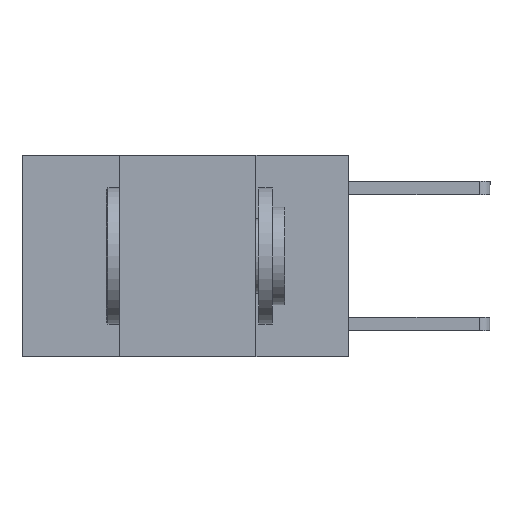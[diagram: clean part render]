
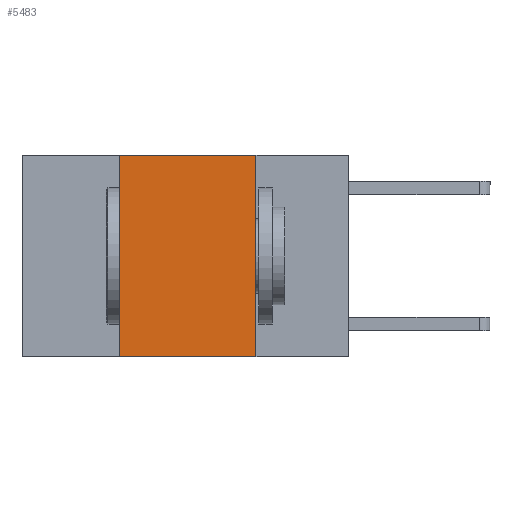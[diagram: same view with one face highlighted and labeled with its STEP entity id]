
A CAD part, left-side view. The second image highlights one B-rep face of the part: STEP entity #5483.
In plain terms, the highlighted planar face has unit normal (-1, 0, 0).
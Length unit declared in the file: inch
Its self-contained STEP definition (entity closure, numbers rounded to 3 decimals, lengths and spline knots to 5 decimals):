
#61 = ORIENTED_EDGE ( 'NONE', *, *, #5642, .F. ) ;
#530 = DIRECTION ( 'NONE',  ( 0., 0., -1. ) ) ;
#706 = LINE ( 'NONE', #3466, #3795 ) ;
#716 = CARTESIAN_POINT ( 'NONE',  ( 0., 0.42, 0. ) ) ;
#812 = VERTEX_POINT ( 'NONE', #1361 ) ;
#1120 = CARTESIAN_POINT ( 'NONE',  ( 0., 0.17, -0.37 ) ) ;
#1247 = LINE ( 'NONE', #4108, #3077 ) ;
#1333 = AXIS2_PLACEMENT_3D ( 'NONE', #3973, #8892, #530 ) ;
#1361 = CARTESIAN_POINT ( 'NONE',  ( 0., 0.42, -0.37 ) ) ;
#1599 = ORIENTED_EDGE ( 'NONE', *, *, #5420, .F. ) ;
#1929 = LINE ( 'NONE', #4697, #6848 ) ;
#2064 = VERTEX_POINT ( 'NONE', #1120 ) ;
#2792 = DIRECTION ( 'NONE',  ( 0., -1., 0. ) ) ;
#3077 = VECTOR ( 'NONE', #4789, 39.37008 ) ;
#3298 = CARTESIAN_POINT ( 'NONE',  ( 0., 0.17, 0. ) ) ;
#3466 = CARTESIAN_POINT ( 'NONE',  ( 0., 0.6, -0.37 ) ) ;
#3509 = LINE ( 'NONE', #5690, #5982 ) ;
#3795 = VECTOR ( 'NONE', #2792, 39.37008 ) ;
#3973 = CARTESIAN_POINT ( 'NONE',  ( 0., 0.6, 0. ) ) ;
#4108 = CARTESIAN_POINT ( 'NONE',  ( 0., 0.17, 0. ) ) ;
#4154 = DIRECTION ( 'NONE',  ( 0., -1., 0. ) ) ;
#4661 = FACE_OUTER_BOUND ( 'NONE', #7631, .T. ) ;
#4697 = CARTESIAN_POINT ( 'NONE',  ( 0., 0.42, 0. ) ) ;
#4789 = DIRECTION ( 'NONE',  ( 0., 0., -1. ) ) ;
#4960 = ORIENTED_EDGE ( 'NONE', *, *, #5509, .F. ) ;
#5420 = EDGE_CURVE ( 'NONE', #7531, #2064, #1247, .T. ) ;
#5483 = ADVANCED_FACE ( 'NONE', ( #4661 ), #8162, .F. ) ;
#5509 = EDGE_CURVE ( 'NONE', #812, #7651, #1929, .T. ) ;
#5642 = EDGE_CURVE ( 'NONE', #7651, #7531, #3509, .T. ) ;
#5643 = EDGE_CURVE ( 'NONE', #812, #2064, #706, .T. ) ;
#5690 = CARTESIAN_POINT ( 'NONE',  ( 0., 0.6, 0. ) ) ;
#5982 = VECTOR ( 'NONE', #4154, 39.37008 ) ;
#6170 = ORIENTED_EDGE ( 'NONE', *, *, #5643, .T. ) ;
#6848 = VECTOR ( 'NONE', #7475, 39.37008 ) ;
#7475 = DIRECTION ( 'NONE',  ( 0., 0., 1. ) ) ;
#7531 = VERTEX_POINT ( 'NONE', #3298 ) ;
#7631 = EDGE_LOOP ( 'NONE', ( #1599, #61, #4960, #6170 ) ) ;
#7651 = VERTEX_POINT ( 'NONE', #716 ) ;
#8162 = PLANE ( 'NONE',  #1333 ) ;
#8892 = DIRECTION ( 'NONE',  ( 1., 0., 0. ) ) ;
